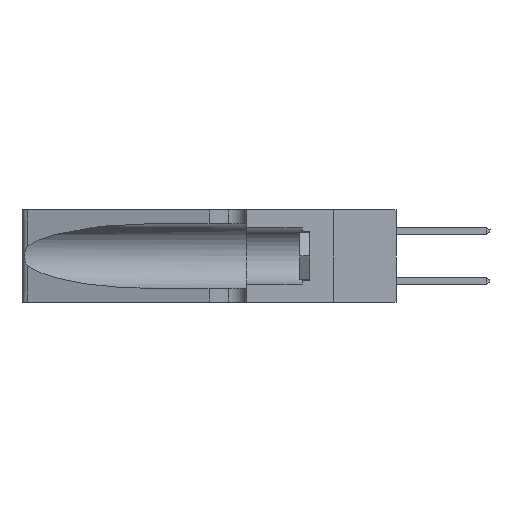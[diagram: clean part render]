
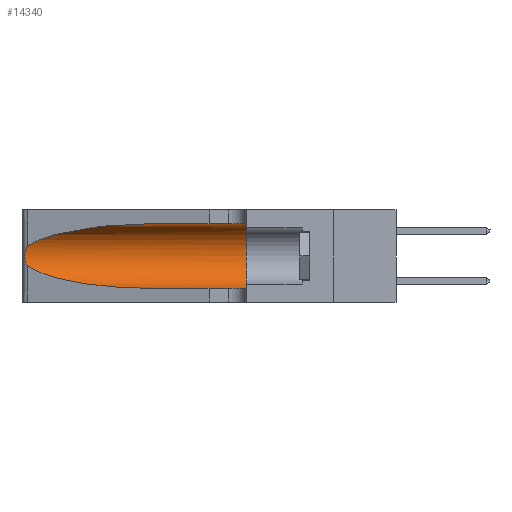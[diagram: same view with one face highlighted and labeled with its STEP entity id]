
A CAD part, left-side view. The second image highlights one B-rep face of the part: STEP entity #14340.
In plain terms, the highlighted cylindrical face has radius 3.308 mm (diameter 6.617 mm), a partial arc.
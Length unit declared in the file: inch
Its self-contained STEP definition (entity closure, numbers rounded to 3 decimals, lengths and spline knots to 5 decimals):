
#362 = CARTESIAN_POINT ( 'NONE',  ( 0.25487, 1.22718, 0.22369 ) ) ;
#891 = EDGE_CURVE ( 'NONE', #1419, #6277, #15378, .T. ) ;
#1104 = CARTESIAN_POINT ( 'NONE',  ( 0.25639, 1.23184, 0.21858 ) ) ;
#1106 = ORIENTED_EDGE ( 'NONE', *, *, #11177, .T. ) ;
#1166 = CARTESIAN_POINT ( 'NONE',  ( 0.26075, 1.23896, 0.178 ) ) ;
#1181 = ORIENTED_EDGE ( 'NONE', *, *, #18553, .T. ) ;
#1419 = VERTEX_POINT ( 'NONE', #362 ) ;
#1781 =( BOUNDED_CURVE ( )  B_SPLINE_CURVE ( 3, ( #4121, #2639, #5513, #18572 ),
 .UNSPECIFIED., .F., .F. ) 
 B_SPLINE_CURVE_WITH_KNOTS ( ( 4, 4 ),
 ( 3.44316, 4.71239 ),
 .UNSPECIFIED. ) 
 CURVE ( )  GEOMETRIC_REPRESENTATION_ITEM ( )  RATIONAL_B_SPLINE_CURVE ( ( 1., 0.87, 0.87, 1. ) ) 
 REPRESENTATION_ITEM ( '' )  );
#1960 = CARTESIAN_POINT ( 'NONE',  ( 0.25487, 1.22718, 0.22369 ) ) ;
#1967 = CARTESIAN_POINT ( 'NONE',  ( 0.25555, 1.22993, 0.14849 ) ) ;
#2283 = VERTEX_POINT ( 'NONE', #16283 ) ;
#2639 = CARTESIAN_POINT ( 'NONE',  ( 0.2373, 1.15595, 0.08982 ) ) ;
#2686 = CARTESIAN_POINT ( 'NONE',  ( 0.25487, 1.22718, 0.14631 ) ) ;
#2961 = EDGE_CURVE ( 'NONE', #6277, #15789, #1781, .T. ) ;
#2987 = AXIS2_PLACEMENT_3D ( 'NONE', #3065, #16285, #17736 ) ;
#3065 = CARTESIAN_POINT ( 'NONE',  ( 0.1305, 0.35, 0.185 ) ) ;
#4121 = CARTESIAN_POINT ( 'NONE',  ( 0.25487, 1.22718, 0.14631 ) ) ;
#4259 = CARTESIAN_POINT ( 'NONE',  ( 0.1305, 1.61858, 0.185 ) ) ;
#4544 = LINE ( 'NONE', #8741, #14132 ) ;
#4726 = CARTESIAN_POINT ( 'NONE',  ( 0.18966, 0.96281, 0.31525 ) ) ;
#5268 = EDGE_LOOP ( 'NONE', ( #1106, #12280, #11765, #1181, #9134, #12944 ) ) ;
#5513 = CARTESIAN_POINT ( 'NONE',  ( 0.18966, 0.96281, 0.05475 ) ) ;
#5575 = CARTESIAN_POINT ( 'NONE',  ( 0.25787, 1.23484, 0.2124 ) ) ;
#6141 = CARTESIAN_POINT ( 'NONE',  ( 0.25639, 1.23186, 0.15144 ) ) ;
#6277 = VERTEX_POINT ( 'NONE', #2686 ) ;
#7366 = CARTESIAN_POINT ( 'NONE',  ( 0.26017, 1.23833, 0.17102 ) ) ;
#7948 = CARTESIAN_POINT ( 'NONE',  ( 0.25487, 1.22718, 0.14631 ) ) ;
#8468 = CARTESIAN_POINT ( 'NONE',  ( 0.25854, 1.2359, 0.20912 ) ) ;
#8741 = CARTESIAN_POINT ( 'NONE',  ( 0.1305, 1.61858, 0.31525 ) ) ;
#9022 = CARTESIAN_POINT ( 'NONE',  ( 0.2373, 1.15595, 0.28018 ) ) ;
#9080 = CARTESIAN_POINT ( 'NONE',  ( 0.1305, 0.72297, 0.31525 ) ) ;
#9134 = ORIENTED_EDGE ( 'NONE', *, *, #15456, .F. ) ;
#9139 = LINE ( 'NONE', #18902, #9375 ) ;
#9375 = VECTOR ( 'NONE', #14517, 39.37008 ) ;
#10130 = CIRCLE ( 'NONE', #2987, 0.13025 ) ;
#11177 = EDGE_CURVE ( 'NONE', #2283, #1419, #15668, .T. ) ;
#11460 = CARTESIAN_POINT ( 'NONE',  ( 0.26018, 1.23835, 0.19895 ) ) ;
#11765 = ORIENTED_EDGE ( 'NONE', *, *, #2961, .T. ) ;
#12280 = ORIENTED_EDGE ( 'NONE', *, *, #891, .T. ) ;
#12474 = CARTESIAN_POINT ( 'NONE',  ( 0.25487, 1.22718, 0.22369 ) ) ;
#12578 = CARTESIAN_POINT ( 'NONE',  ( 0.1305, 0.35, 0.05475 ) ) ;
#12944 = ORIENTED_EDGE ( 'NONE', *, *, #18587, .F. ) ;
#13394 = CARTESIAN_POINT ( 'NONE',  ( 0.1305, 0.72297, 0.05475 ) ) ;
#14132 = VECTOR ( 'NONE', #17399, 39.37008 ) ;
#14340 = ADVANCED_FACE ( 'NONE', ( #17017 ), #16105, .F. ) ;
#14465 = DIRECTION ( 'NONE',  ( 0., -1., 0. ) ) ;
#14478 = AXIS2_PLACEMENT_3D ( 'NONE', #4259, #14465, #17837 ) ;
#14517 = DIRECTION ( 'NONE',  ( 0., -1., 0. ) ) ;
#15378 = B_SPLINE_CURVE_WITH_KNOTS ( 'NONE', 3,
 ( #12474, #17010, #1104, #5575, #8468, #11460, #15595, #1166, #7366, #17745, #17812, #6141, #1967, #7948 ),
 .UNSPECIFIED., .F., .F.,
 ( 4, 2, 2, 2, 2, 2, 4 ),
 ( 0., 0.00027, 0.00053, 0.00107, 0.0016, 0.00187, 0.00214 ),
 .UNSPECIFIED. ) ;
#15456 = EDGE_CURVE ( 'NONE', #18218, #17153, #10130, .T. ) ;
#15595 = CARTESIAN_POINT ( 'NONE',  ( 0.26075, 1.23896, 0.19203 ) ) ;
#15668 =( BOUNDED_CURVE ( )  B_SPLINE_CURVE ( 3, ( #9080, #4726, #9022, #1960 ),
 .UNSPECIFIED., .F., .T. ) 
 B_SPLINE_CURVE_WITH_KNOTS ( ( 4, 4 ),
 ( 1.5708, 2.84003 ),
 .UNSPECIFIED. ) 
 CURVE ( )  GEOMETRIC_REPRESENTATION_ITEM ( )  RATIONAL_B_SPLINE_CURVE ( ( 1., 0.87, 0.87, 1. ) ) 
 REPRESENTATION_ITEM ( '' )  );
#15789 = VERTEX_POINT ( 'NONE', #13394 ) ;
#16105 = CYLINDRICAL_SURFACE ( 'NONE', #14478, 0.13025 ) ;
#16283 = CARTESIAN_POINT ( 'NONE',  ( 0.1305, 0.72297, 0.31525 ) ) ;
#16285 = DIRECTION ( 'NONE',  ( 0., 1., 0. ) ) ;
#16327 = CARTESIAN_POINT ( 'NONE',  ( 0.1305, 0.35, 0.31525 ) ) ;
#17010 = CARTESIAN_POINT ( 'NONE',  ( 0.25555, 1.22994, 0.2215 ) ) ;
#17017 = FACE_OUTER_BOUND ( 'NONE', #5268, .T. ) ;
#17153 = VERTEX_POINT ( 'NONE', #12578 ) ;
#17399 = DIRECTION ( 'NONE',  ( 0., -1., 0. ) ) ;
#17736 = DIRECTION ( 'NONE',  ( 0., 0., 1. ) ) ;
#17745 = CARTESIAN_POINT ( 'NONE',  ( 0.25856, 1.23593, 0.16098 ) ) ;
#17812 = CARTESIAN_POINT ( 'NONE',  ( 0.25789, 1.23486, 0.15765 ) ) ;
#17837 = DIRECTION ( 'NONE',  ( 0., 0., -1. ) ) ;
#18218 = VERTEX_POINT ( 'NONE', #16327 ) ;
#18553 = EDGE_CURVE ( 'NONE', #15789, #17153, #9139, .T. ) ;
#18572 = CARTESIAN_POINT ( 'NONE',  ( 0.1305, 0.72297, 0.05475 ) ) ;
#18587 = EDGE_CURVE ( 'NONE', #2283, #18218, #4544, .T. ) ;
#18902 = CARTESIAN_POINT ( 'NONE',  ( 0.1305, 1.61858, 0.05475 ) ) ;
